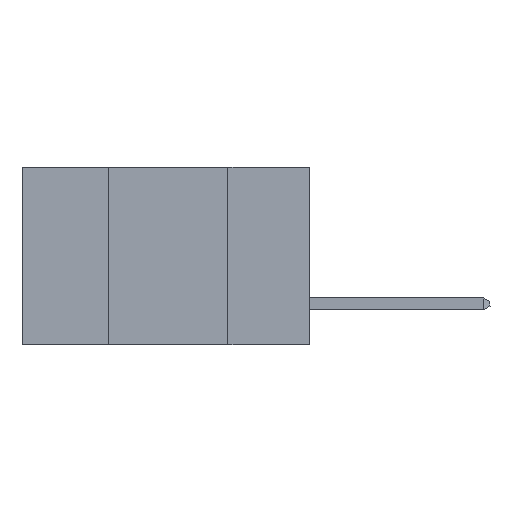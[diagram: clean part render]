
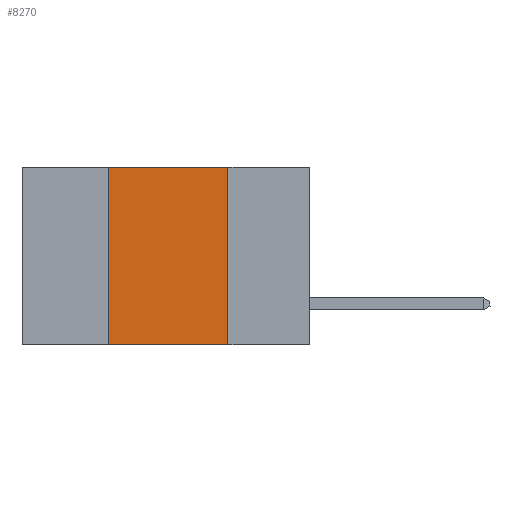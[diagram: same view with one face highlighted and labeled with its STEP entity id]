
A CAD part, left-side view. The second image highlights one B-rep face of the part: STEP entity #8270.
In plain terms, the highlighted planar face has unit normal (-1, 0, 0).
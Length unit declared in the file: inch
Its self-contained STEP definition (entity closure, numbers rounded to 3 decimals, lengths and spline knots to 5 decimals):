
#115 = EDGE_CURVE ( 'NONE', #2836, #2733, #9560, .T. ) ;
#142 = CARTESIAN_POINT ( 'NONE',  ( 0., 0.6, -0.37 ) ) ;
#356 = ORIENTED_EDGE ( 'NONE', *, *, #8355, .F. ) ;
#730 = CARTESIAN_POINT ( 'NONE',  ( 0., 0.6, 0. ) ) ;
#1582 = CARTESIAN_POINT ( 'NONE',  ( 0., 0.42, 0. ) ) ;
#2111 = VECTOR ( 'NONE', #8133, 39.37008 ) ;
#2222 = LINE ( 'NONE', #3367, #2111 ) ;
#2339 = VERTEX_POINT ( 'NONE', #4768 ) ;
#2411 = DIRECTION ( 'NONE',  ( 1., 0., 0. ) ) ;
#2609 = VECTOR ( 'NONE', #5059, 39.37008 ) ;
#2733 = VERTEX_POINT ( 'NONE', #10615 ) ;
#2836 = VERTEX_POINT ( 'NONE', #9763 ) ;
#3250 = DIRECTION ( 'NONE',  ( 0., 0., -1. ) ) ;
#3367 = CARTESIAN_POINT ( 'NONE',  ( 0., 0.17, 0. ) ) ;
#3548 = EDGE_LOOP ( 'NONE', ( #356, #10148, #7474, #9027 ) ) ;
#4026 = PLANE ( 'NONE',  #7423 ) ;
#4768 = CARTESIAN_POINT ( 'NONE',  ( 0., 0.17, 0. ) ) ;
#5059 = DIRECTION ( 'NONE',  ( 0., -1., 0. ) ) ;
#5301 = VECTOR ( 'NONE', #5898, 39.37008 ) ;
#5898 = DIRECTION ( 'NONE',  ( 0., -1., 0. ) ) ;
#6112 = FACE_OUTER_BOUND ( 'NONE', #3548, .T. ) ;
#6530 = EDGE_CURVE ( 'NONE', #9454, #2339, #10332, .T. ) ;
#6837 = VECTOR ( 'NONE', #7353, 39.37008 ) ;
#7353 = DIRECTION ( 'NONE',  ( 0., 0., 1. ) ) ;
#7423 = AXIS2_PLACEMENT_3D ( 'NONE', #730, #2411, #3250 ) ;
#7474 = ORIENTED_EDGE ( 'NONE', *, *, #10357, .F. ) ;
#8133 = DIRECTION ( 'NONE',  ( 0., 0., -1. ) ) ;
#8242 = CARTESIAN_POINT ( 'NONE',  ( 0., 0.6, 0. ) ) ;
#8270 = ADVANCED_FACE ( 'NONE', ( #6112 ), #4026, .F. ) ;
#8355 = EDGE_CURVE ( 'NONE', #2339, #2733, #2222, .T. ) ;
#9027 = ORIENTED_EDGE ( 'NONE', *, *, #115, .T. ) ;
#9454 = VERTEX_POINT ( 'NONE', #10499 ) ;
#9560 = LINE ( 'NONE', #142, #2609 ) ;
#9763 = CARTESIAN_POINT ( 'NONE',  ( 0., 0.42, -0.37 ) ) ;
#9935 = LINE ( 'NONE', #1582, #6837 ) ;
#10148 = ORIENTED_EDGE ( 'NONE', *, *, #6530, .F. ) ;
#10332 = LINE ( 'NONE', #8242, #5301 ) ;
#10357 = EDGE_CURVE ( 'NONE', #2836, #9454, #9935, .T. ) ;
#10499 = CARTESIAN_POINT ( 'NONE',  ( 0., 0.42, 0. ) ) ;
#10615 = CARTESIAN_POINT ( 'NONE',  ( 0., 0.17, -0.37 ) ) ;
